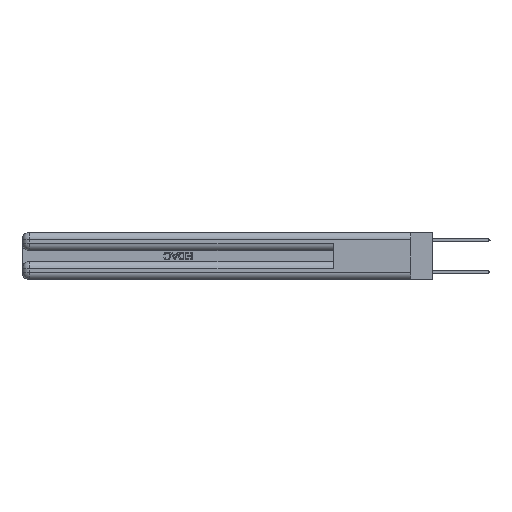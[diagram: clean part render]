
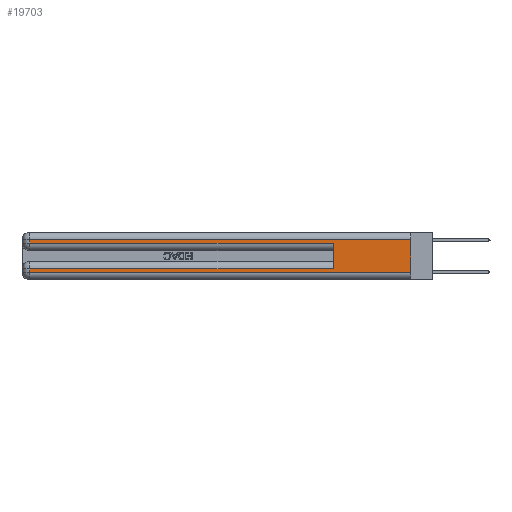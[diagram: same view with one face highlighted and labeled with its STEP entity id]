
A CAD part, left-side view. The second image highlights one B-rep face of the part: STEP entity #19703.
In plain terms, the highlighted planar face has unit normal (-1, 0, 0).
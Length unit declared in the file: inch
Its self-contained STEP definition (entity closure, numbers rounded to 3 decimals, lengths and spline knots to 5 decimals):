
#252 = ORIENTED_EDGE ( 'NONE', *, *, #26755, .T. ) ;
#967 = CARTESIAN_POINT ( 'NONE',  ( 0., 0.6, 0.285 ) ) ;
#1102 = CARTESIAN_POINT ( 'NONE',  ( 0., 0., 0.31 ) ) ;
#1133 = CARTESIAN_POINT ( 'NONE',  ( 0., 0., 0.37 ) ) ;
#1146 = CARTESIAN_POINT ( 'NONE',  ( 0., 0., 0.06 ) ) ;
#1538 = VERTEX_POINT ( 'NONE', #29662 ) ;
#2154 = FACE_OUTER_BOUND ( 'NONE', #2843, .T. ) ;
#2265 = ORIENTED_EDGE ( 'NONE', *, *, #29960, .T. ) ;
#2843 = EDGE_LOOP ( 'NONE', ( #8469, #27559, #27920, #2265, #22410, #252, #31639, #20946 ) ) ;
#3082 = CARTESIAN_POINT ( 'NONE',  ( 0., 0., 0.31 ) ) ;
#3973 = DIRECTION ( 'NONE',  ( 0., 0., -1. ) ) ;
#4381 = CARTESIAN_POINT ( 'NONE',  ( 0., 0., 0.37 ) ) ;
#4562 = CARTESIAN_POINT ( 'NONE',  ( 0., 0., 0.06 ) ) ;
#5281 = LINE ( 'NONE', #3082, #12792 ) ;
#6577 = VECTOR ( 'NONE', #14978, 39.37008 ) ;
#6606 = LINE ( 'NONE', #22997, #35595 ) ;
#7294 = CARTESIAN_POINT ( 'NONE',  ( 0., 0., 0.285 ) ) ;
#8469 = ORIENTED_EDGE ( 'NONE', *, *, #33242, .F. ) ;
#9779 = VECTOR ( 'NONE', #29788, 39.37008 ) ;
#9834 = VERTEX_POINT ( 'NONE', #16596 ) ;
#12031 = CARTESIAN_POINT ( 'NONE',  ( 0., 0.6, 0.145 ) ) ;
#12564 = EDGE_CURVE ( 'NONE', #13546, #9834, #14701, .T. ) ;
#12792 = VECTOR ( 'NONE', #28391, 39.37008 ) ;
#13546 = VERTEX_POINT ( 'NONE', #16374 ) ;
#14298 = EDGE_CURVE ( 'NONE', #30791, #1538, #6606, .T. ) ;
#14393 = DIRECTION ( 'NONE',  ( 0., 0., -1. ) ) ;
#14459 = VERTEX_POINT ( 'NONE', #1146 ) ;
#14701 = LINE ( 'NONE', #17226, #23077 ) ;
#14978 = DIRECTION ( 'NONE',  ( 0., 1., 0. ) ) ;
#15103 = VERTEX_POINT ( 'NONE', #1102 ) ;
#15411 = CARTESIAN_POINT ( 'NONE',  ( 0., 0.6, 0.085 ) ) ;
#16150 = VECTOR ( 'NONE', #29601, 39.37008 ) ;
#16251 = CARTESIAN_POINT ( 'NONE',  ( 0., 2.94, 0.085 ) ) ;
#16374 = CARTESIAN_POINT ( 'NONE',  ( 0., 2.94, 0.31 ) ) ;
#16596 = CARTESIAN_POINT ( 'NONE',  ( 0., 2.94, 0.285 ) ) ;
#16784 = LINE ( 'NONE', #12031, #33441 ) ;
#17129 = AXIS2_PLACEMENT_3D ( 'NONE', #1133, #20905, #3973 ) ;
#17226 = CARTESIAN_POINT ( 'NONE',  ( 0., 2.94, 0.37 ) ) ;
#18045 = PLANE ( 'NONE',  #17129 ) ;
#18376 = VECTOR ( 'NONE', #24279, 39.37008 ) ;
#18956 = EDGE_CURVE ( 'NONE', #23598, #35060, #16784, .T. ) ;
#19703 = ADVANCED_FACE ( 'NONE', ( #2154 ), #18045, .F. ) ;
#19862 = LINE ( 'NONE', #34574, #6577 ) ;
#20161 = LINE ( 'NONE', #4562, #18376 ) ;
#20905 = DIRECTION ( 'NONE',  ( 1., 0., 0. ) ) ;
#20946 = ORIENTED_EDGE ( 'NONE', *, *, #21875, .T. ) ;
#21875 = EDGE_CURVE ( 'NONE', #1538, #14459, #20161, .T. ) ;
#22410 = ORIENTED_EDGE ( 'NONE', *, *, #18956, .F. ) ;
#22997 = CARTESIAN_POINT ( 'NONE',  ( 0., 2.94, 0.37 ) ) ;
#23077 = VECTOR ( 'NONE', #14393, 39.37008 ) ;
#23598 = VERTEX_POINT ( 'NONE', #15411 ) ;
#24279 = DIRECTION ( 'NONE',  ( 0., -1., 0. ) ) ;
#26755 = EDGE_CURVE ( 'NONE', #23598, #30791, #19862, .T. ) ;
#27559 = ORIENTED_EDGE ( 'NONE', *, *, #31004, .T. ) ;
#27920 = ORIENTED_EDGE ( 'NONE', *, *, #12564, .T. ) ;
#28391 = DIRECTION ( 'NONE',  ( 0., 1., 0. ) ) ;
#28583 = DIRECTION ( 'NONE',  ( 0., 0., -1. ) ) ;
#28833 = DIRECTION ( 'NONE',  ( 0., 0., 1. ) ) ;
#29601 = DIRECTION ( 'NONE',  ( 0., 0., -1. ) ) ;
#29662 = CARTESIAN_POINT ( 'NONE',  ( 0., 2.94, 0.06 ) ) ;
#29788 = DIRECTION ( 'NONE',  ( 0., -1., 0. ) ) ;
#29960 = EDGE_CURVE ( 'NONE', #9834, #35060, #31307, .T. ) ;
#30171 = LINE ( 'NONE', #4381, #16150 ) ;
#30791 = VERTEX_POINT ( 'NONE', #16251 ) ;
#31004 = EDGE_CURVE ( 'NONE', #15103, #13546, #5281, .T. ) ;
#31307 = LINE ( 'NONE', #7294, #9779 ) ;
#31639 = ORIENTED_EDGE ( 'NONE', *, *, #14298, .T. ) ;
#33242 = EDGE_CURVE ( 'NONE', #15103, #14459, #30171, .T. ) ;
#33441 = VECTOR ( 'NONE', #28833, 39.37008 ) ;
#34574 = CARTESIAN_POINT ( 'NONE',  ( 0., 0., 0.085 ) ) ;
#35060 = VERTEX_POINT ( 'NONE', #967 ) ;
#35595 = VECTOR ( 'NONE', #28583, 39.37008 ) ;
